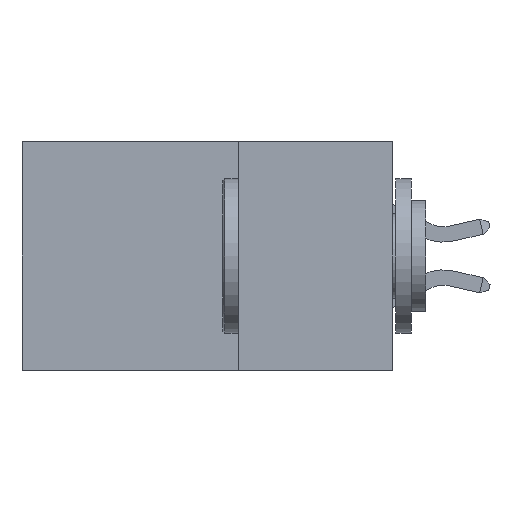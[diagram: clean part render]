
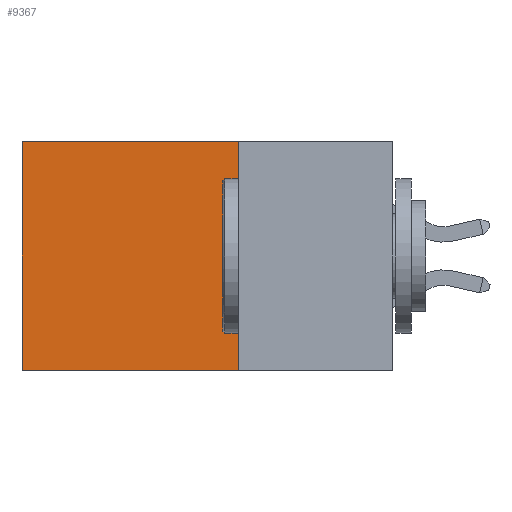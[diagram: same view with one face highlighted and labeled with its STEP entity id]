
A CAD part, left-side view. The second image highlights one B-rep face of the part: STEP entity #9367.
In plain terms, the highlighted planar face has unit normal (-1, 0, 0).
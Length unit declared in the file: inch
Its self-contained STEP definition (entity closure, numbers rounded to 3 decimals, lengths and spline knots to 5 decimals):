
#268 = VECTOR ( 'NONE', #18291, 39.37008 ) ;
#621 = PLANE ( 'NONE',  #18708 ) ;
#996 = EDGE_CURVE ( 'NONE', #16682, #16944, #7060, .T. ) ;
#1152 = DIRECTION ( 'NONE',  ( 1., 0., 0. ) ) ;
#2385 = DIRECTION ( 'NONE',  ( 0., 0., -1. ) ) ;
#2724 = CARTESIAN_POINT ( 'NONE',  ( 0.2875, 0.25, 0. ) ) ;
#5185 = ORIENTED_EDGE ( 'NONE', *, *, #996, .F. ) ;
#5276 = CARTESIAN_POINT ( 'NONE',  ( 0.2875, 0.6, -0.37 ) ) ;
#5532 = VERTEX_POINT ( 'NONE', #10156 ) ;
#5589 = VECTOR ( 'NONE', #8631, 39.37008 ) ;
#5960 = VECTOR ( 'NONE', #24031, 39.37008 ) ;
#6497 = CARTESIAN_POINT ( 'NONE',  ( 0.2875, 0.25, -0.37 ) ) ;
#6779 = VECTOR ( 'NONE', #17717, 39.37008 ) ;
#7060 = LINE ( 'NONE', #6497, #268 ) ;
#8631 = DIRECTION ( 'NONE',  ( 0., 1., 0. ) ) ;
#9296 = EDGE_CURVE ( 'NONE', #25023, #5532, #21744, .T. ) ;
#9367 = ADVANCED_FACE ( 'NONE', ( #16773 ), #621, .F. ) ;
#10156 = CARTESIAN_POINT ( 'NONE',  ( 0.2875, 0.6, 0. ) ) ;
#10343 = EDGE_LOOP ( 'NONE', ( #12904, #5185, #18271, #15410 ) ) ;
#10989 = CARTESIAN_POINT ( 'NONE',  ( 0.2875, 0.25, -0.37 ) ) ;
#11966 = LINE ( 'NONE', #19486, #6779 ) ;
#12904 = ORIENTED_EDGE ( 'NONE', *, *, #21309, .T. ) ;
#15410 = ORIENTED_EDGE ( 'NONE', *, *, #9296, .T. ) ;
#16682 = VERTEX_POINT ( 'NONE', #10989 ) ;
#16773 = FACE_OUTER_BOUND ( 'NONE', #10343, .T. ) ;
#16944 = VERTEX_POINT ( 'NONE', #5276 ) ;
#17717 = DIRECTION ( 'NONE',  ( 0., 0., -1. ) ) ;
#18271 = ORIENTED_EDGE ( 'NONE', *, *, #21156, .F. ) ;
#18291 = DIRECTION ( 'NONE',  ( 0., 1., 0. ) ) ;
#18491 = CARTESIAN_POINT ( 'NONE',  ( 0.2875, 0.25, 0. ) ) ;
#18708 = AXIS2_PLACEMENT_3D ( 'NONE', #2724, #1152, #2385 ) ;
#19486 = CARTESIAN_POINT ( 'NONE',  ( 0.2875, 0.25, 0. ) ) ;
#20819 = LINE ( 'NONE', #23951, #5960 ) ;
#21156 = EDGE_CURVE ( 'NONE', #25023, #16682, #11966, .T. ) ;
#21173 = CARTESIAN_POINT ( 'NONE',  ( 0.2875, 0.25, 0. ) ) ;
#21309 = EDGE_CURVE ( 'NONE', #5532, #16944, #20819, .T. ) ;
#21744 = LINE ( 'NONE', #18491, #5589 ) ;
#23951 = CARTESIAN_POINT ( 'NONE',  ( 0.2875, 0.6, 0. ) ) ;
#24031 = DIRECTION ( 'NONE',  ( 0., 0., -1. ) ) ;
#25023 = VERTEX_POINT ( 'NONE', #21173 ) ;
